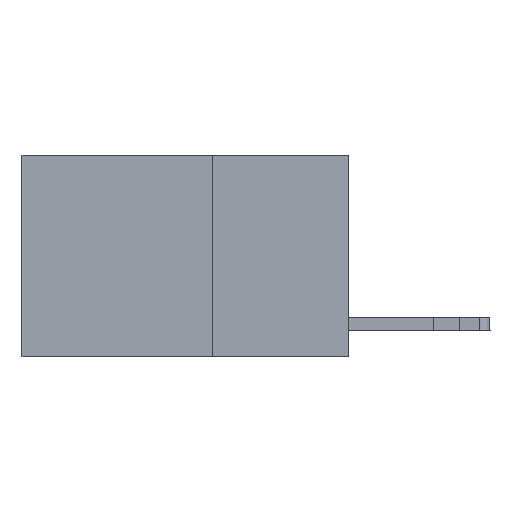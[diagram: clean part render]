
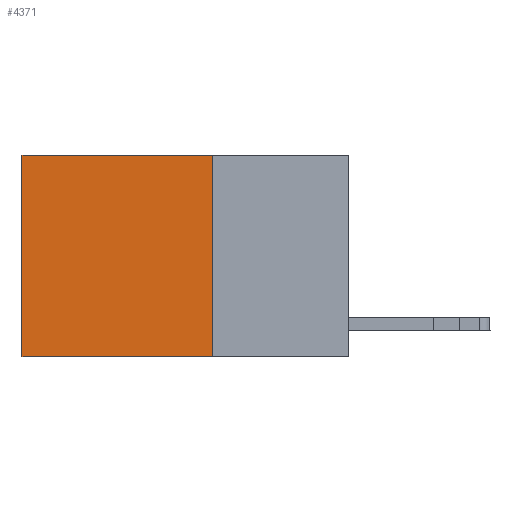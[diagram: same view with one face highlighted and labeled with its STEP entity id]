
A CAD part, left-side view. The second image highlights one B-rep face of the part: STEP entity #4371.
In plain terms, the highlighted planar face has unit normal (-1, 0, 0).
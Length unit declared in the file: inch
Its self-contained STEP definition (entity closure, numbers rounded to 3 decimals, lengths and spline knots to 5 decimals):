
#252 = CARTESIAN_POINT ( 'NONE',  ( 0.2625, 0.6, 0. ) ) ;
#864 = CARTESIAN_POINT ( 'NONE',  ( 0.2625, 0.6, -0.37 ) ) ;
#1865 = EDGE_CURVE ( 'NONE', #14889, #12282, #13448, .T. ) ;
#2026 = ORIENTED_EDGE ( 'NONE', *, *, #1865, .F. ) ;
#2653 = CARTESIAN_POINT ( 'NONE',  ( 0.2625, 0.25, 0. ) ) ;
#4204 = VECTOR ( 'NONE', #7746, 39.37008 ) ;
#4311 = ORIENTED_EDGE ( 'NONE', *, *, #17980, .F. ) ;
#4334 = PLANE ( 'NONE',  #5051 ) ;
#4371 = ADVANCED_FACE ( 'NONE', ( #20724 ), #4334, .F. ) ;
#4679 = DIRECTION ( 'NONE',  ( 0., 0., -1. ) ) ;
#5051 = AXIS2_PLACEMENT_3D ( 'NONE', #21093, #8305, #4679 ) ;
#6531 = CARTESIAN_POINT ( 'NONE',  ( 0.2625, 0.25, -0.37 ) ) ;
#6590 = ORIENTED_EDGE ( 'NONE', *, *, #10214, .T. ) ;
#7746 = DIRECTION ( 'NONE',  ( 0., 0., -1. ) ) ;
#8305 = DIRECTION ( 'NONE',  ( 1., 0., 0. ) ) ;
#8937 = LINE ( 'NONE', #6531, #17316 ) ;
#9342 = DIRECTION ( 'NONE',  ( 0., 0., -1. ) ) ;
#10214 = EDGE_CURVE ( 'NONE', #11424, #14702, #20198, .T. ) ;
#10236 = VECTOR ( 'NONE', #10442, 39.37008 ) ;
#10442 = DIRECTION ( 'NONE',  ( 0., 1., 0. ) ) ;
#10582 = EDGE_LOOP ( 'NONE', ( #6590, #4311, #2026, #17432 ) ) ;
#11424 = VERTEX_POINT ( 'NONE', #11929 ) ;
#11929 = CARTESIAN_POINT ( 'NONE',  ( 0.2625, 0.6, 0. ) ) ;
#12247 = EDGE_CURVE ( 'NONE', #14889, #11424, #23503, .T. ) ;
#12282 = VERTEX_POINT ( 'NONE', #12665 ) ;
#12665 = CARTESIAN_POINT ( 'NONE',  ( 0.2625, 0.25, -0.37 ) ) ;
#13448 = LINE ( 'NONE', #17537, #4204 ) ;
#14094 = DIRECTION ( 'NONE',  ( 0., 1., 0. ) ) ;
#14404 = CARTESIAN_POINT ( 'NONE',  ( 0.2625, 0.25, 0. ) ) ;
#14702 = VERTEX_POINT ( 'NONE', #864 ) ;
#14889 = VERTEX_POINT ( 'NONE', #2653 ) ;
#17316 = VECTOR ( 'NONE', #14094, 39.37008 ) ;
#17432 = ORIENTED_EDGE ( 'NONE', *, *, #12247, .T. ) ;
#17537 = CARTESIAN_POINT ( 'NONE',  ( 0.2625, 0.25, 0. ) ) ;
#17980 = EDGE_CURVE ( 'NONE', #12282, #14702, #8937, .T. ) ;
#20198 = LINE ( 'NONE', #252, #23208 ) ;
#20724 = FACE_OUTER_BOUND ( 'NONE', #10582, .T. ) ;
#21093 = CARTESIAN_POINT ( 'NONE',  ( 0.2625, 0.25, 0. ) ) ;
#23208 = VECTOR ( 'NONE', #9342, 39.37008 ) ;
#23503 = LINE ( 'NONE', #14404, #10236 ) ;
